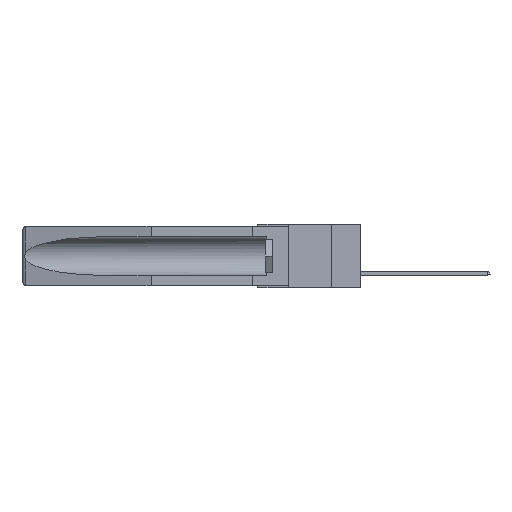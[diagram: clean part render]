
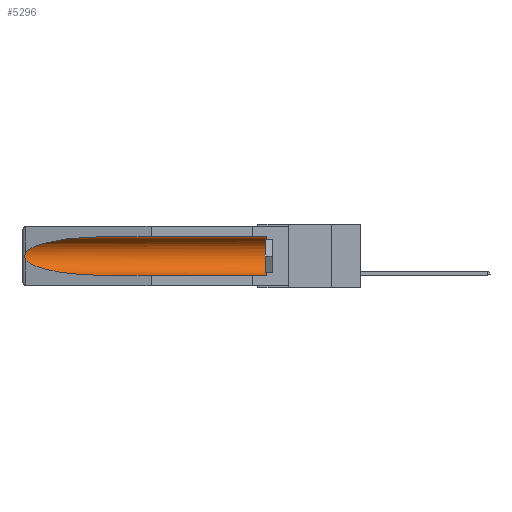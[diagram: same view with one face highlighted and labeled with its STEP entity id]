
A CAD part, left-side view. The second image highlights one B-rep face of the part: STEP entity #5296.
In plain terms, the highlighted cylindrical face has radius 2.857 mm (diameter 5.715 mm), a partial arc.
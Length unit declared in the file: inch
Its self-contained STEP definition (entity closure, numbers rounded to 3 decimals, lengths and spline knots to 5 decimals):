
#518 = CARTESIAN_POINT ( 'NONE',  ( 0.21114, 1.30732, -0.284 ) ) ;
#670 = CIRCLE ( 'NONE', #5817, 0.1125 ) ;
#956 = CARTESIAN_POINT ( 'NONE',  ( 0.155, 0.126, -0.284 ) ) ;
#993 = VERTEX_POINT ( 'NONE', #8005 ) ;
#1354 = CARTESIAN_POINT ( 'NONE',  ( 0.155, -0.30754, -0.059 ) ) ;
#1749 = VERTEX_POINT ( 'NONE', #1767 ) ;
#1767 = CARTESIAN_POINT ( 'NONE',  ( 0.155, 1.07973, -0.059 ) ) ;
#1793 = CARTESIAN_POINT ( 'NONE',  ( 0.155, 0.126, -0.1715 ) ) ;
#1995 = CARTESIAN_POINT ( 'NONE',  ( 0.155, 0.126, -0.059 ) ) ;
#2160 = CARTESIAN_POINT ( 'NONE',  ( 0.26537, 1.52718, -0.19328 ) ) ;
#2878 =( BOUNDED_CURVE ( )  B_SPLINE_CURVE ( 3, ( #6376, #17252, #5333, #6850 ),
 .UNSPECIFIED., .F., .F. ) 
 B_SPLINE_CURVE_WITH_KNOTS ( ( 4, 4 ),
 ( 4.71239, 6.08839 ),
 .UNSPECIFIED. ) 
 CURVE ( )  GEOMETRIC_REPRESENTATION_ITEM ( )  RATIONAL_B_SPLINE_CURVE ( ( 1., 0.848, 0.848, 1. ) ) 
 REPRESENTATION_ITEM ( '' )  );
#3181 = CARTESIAN_POINT ( 'NONE',  ( 0.26597, 1.5296, -0.19026 ) ) ;
#4115 =( BOUNDED_CURVE ( )  B_SPLINE_CURVE ( 3, ( #2160, #5390, #518, #19266 ),
 .UNSPECIFIED., .F., .F. ) 
 B_SPLINE_CURVE_WITH_KNOTS ( ( 4, 4 ),
 ( 0.1948, 1.5708 ),
 .UNSPECIFIED. ) 
 CURVE ( )  GEOMETRIC_REPRESENTATION_ITEM ( )  RATIONAL_B_SPLINE_CURVE ( ( 1., 0.848, 0.848, 1. ) ) 
 REPRESENTATION_ITEM ( '' )  );
#4818 = CARTESIAN_POINT ( 'NONE',  ( 0.26655, 1.53094, -0.18657 ) ) ;
#4906 = ORIENTED_EDGE ( 'NONE', *, *, #12875, .T. ) ;
#5296 = ADVANCED_FACE ( 'NONE', ( #12248 ), #7650, .F. ) ;
#5333 = CARTESIAN_POINT ( 'NONE',  ( 0.25451, 1.48313, -0.09465 ) ) ;
#5357 = DIRECTION ( 'NONE',  ( 0., 0., 1. ) ) ;
#5366 = AXIS2_PLACEMENT_3D ( 'NONE', #17734, #13094, #5357 ) ;
#5390 = CARTESIAN_POINT ( 'NONE',  ( 0.25451, 1.48313, -0.24835 ) ) ;
#5817 = AXIS2_PLACEMENT_3D ( 'NONE', #1793, #17369, #14112 ) ;
#6376 = CARTESIAN_POINT ( 'NONE',  ( 0.155, 1.07973, -0.059 ) ) ;
#6850 = CARTESIAN_POINT ( 'NONE',  ( 0.26537, 1.52718, -0.14972 ) ) ;
#7204 = DIRECTION ( 'NONE',  ( 0., 1., 0. ) ) ;
#7420 = ORIENTED_EDGE ( 'NONE', *, *, #16338, .F. ) ;
#7529 = ORIENTED_EDGE ( 'NONE', *, *, #18805, .T. ) ;
#7650 = CYLINDRICAL_SURFACE ( 'NONE', #5366, 0.1125 ) ;
#8005 = CARTESIAN_POINT ( 'NONE',  ( 0.155, 1.07973, -0.284 ) ) ;
#8708 = VECTOR ( 'NONE', #7204, 39.37008 ) ;
#8736 = EDGE_CURVE ( 'NONE', #10585, #993, #4115, .T. ) ;
#9460 = CARTESIAN_POINT ( 'NONE',  ( 0.2673, 1.5327, -0.16383 ) ) ;
#9621 = B_SPLINE_CURVE_WITH_KNOTS ( 'NONE', 3,
 ( #11014, #15813, #17135, #9460, #18563, #18638, #14077, #4818, #3181, #17062 ),
 .UNSPECIFIED., .F., .F.,
 ( 4, 2, 2, 2, 4 ),
 ( 0., 0.00029, 0.00058, 0.00087, 0.00117 ),
 .UNSPECIFIED. ) ;
#9900 = EDGE_CURVE ( 'NONE', #16494, #1749, #13816, .T. ) ;
#10585 = VERTEX_POINT ( 'NONE', #10973 ) ;
#10973 = CARTESIAN_POINT ( 'NONE',  ( 0.26537, 1.52718, -0.19328 ) ) ;
#11014 = CARTESIAN_POINT ( 'NONE',  ( 0.26537, 1.52718, -0.14972 ) ) ;
#12248 = FACE_OUTER_BOUND ( 'NONE', #16127, .T. ) ;
#12830 = VECTOR ( 'NONE', #20027, 39.37008 ) ;
#12875 = EDGE_CURVE ( 'NONE', #13080, #10585, #9621, .T. ) ;
#13080 = VERTEX_POINT ( 'NONE', #18188 ) ;
#13094 = DIRECTION ( 'NONE',  ( 0., 1., 0. ) ) ;
#13816 = LINE ( 'NONE', #1354, #12830 ) ;
#14077 = CARTESIAN_POINT ( 'NONE',  ( 0.2673, 1.53269, -0.17917 ) ) ;
#14112 = DIRECTION ( 'NONE',  ( 0., 0., 1. ) ) ;
#14451 = ORIENTED_EDGE ( 'NONE', *, *, #9900, .T. ) ;
#14478 = CARTESIAN_POINT ( 'NONE',  ( 0.155, -0.30754, -0.284 ) ) ;
#15813 = CARTESIAN_POINT ( 'NONE',  ( 0.26597, 1.52961, -0.15275 ) ) ;
#15841 = ORIENTED_EDGE ( 'NONE', *, *, #8736, .T. ) ;
#16127 = EDGE_LOOP ( 'NONE', ( #7529, #4906, #15841, #7420, #19606, #14451 ) ) ;
#16338 = EDGE_CURVE ( 'NONE', #17301, #993, #18921, .T. ) ;
#16494 = VERTEX_POINT ( 'NONE', #1995 ) ;
#16498 = EDGE_CURVE ( 'NONE', #17301, #16494, #670, .T. ) ;
#17062 = CARTESIAN_POINT ( 'NONE',  ( 0.26537, 1.52718, -0.19328 ) ) ;
#17135 = CARTESIAN_POINT ( 'NONE',  ( 0.26654, 1.53092, -0.15636 ) ) ;
#17252 = CARTESIAN_POINT ( 'NONE',  ( 0.21114, 1.30732, -0.059 ) ) ;
#17301 = VERTEX_POINT ( 'NONE', #956 ) ;
#17369 = DIRECTION ( 'NONE',  ( 0., -1., 0. ) ) ;
#17734 = CARTESIAN_POINT ( 'NONE',  ( 0.155, -0.30754, -0.1715 ) ) ;
#18188 = CARTESIAN_POINT ( 'NONE',  ( 0.26537, 1.52718, -0.14972 ) ) ;
#18563 = CARTESIAN_POINT ( 'NONE',  ( 0.2675, 1.53308, -0.16763 ) ) ;
#18638 = CARTESIAN_POINT ( 'NONE',  ( 0.2675, 1.53308, -0.17534 ) ) ;
#18805 = EDGE_CURVE ( 'NONE', #1749, #13080, #2878, .T. ) ;
#18921 = LINE ( 'NONE', #14478, #8708 ) ;
#19266 = CARTESIAN_POINT ( 'NONE',  ( 0.155, 1.07973, -0.284 ) ) ;
#19606 = ORIENTED_EDGE ( 'NONE', *, *, #16498, .T. ) ;
#20027 = DIRECTION ( 'NONE',  ( 0., 1., 0. ) ) ;
